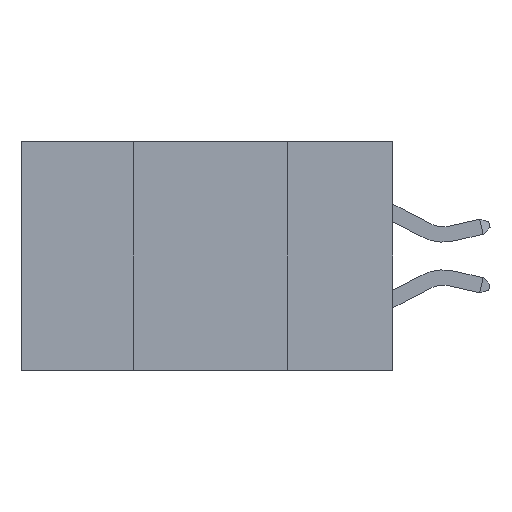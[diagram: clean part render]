
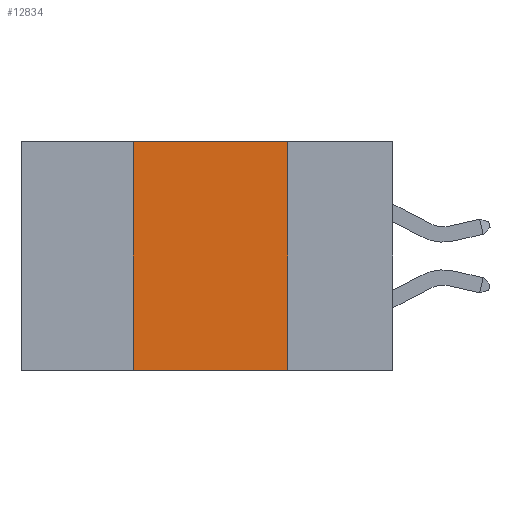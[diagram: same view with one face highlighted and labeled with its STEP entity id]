
A CAD part, left-side view. The second image highlights one B-rep face of the part: STEP entity #12834.
In plain terms, the highlighted planar face has unit normal (-1, 0, 0).
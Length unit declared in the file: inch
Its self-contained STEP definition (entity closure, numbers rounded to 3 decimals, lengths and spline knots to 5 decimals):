
#938 = ORIENTED_EDGE ( 'NONE', *, *, #9733, .T. ) ;
#943 = VECTOR ( 'NONE', #3581, 39.37008 ) ;
#1372 = CARTESIAN_POINT ( 'NONE',  ( 0., 0.6, 0. ) ) ;
#1464 = EDGE_CURVE ( 'NONE', #2867, #10343, #8704, .T. ) ;
#2004 = CARTESIAN_POINT ( 'NONE',  ( 0., 0.42, 0. ) ) ;
#2183 = CARTESIAN_POINT ( 'NONE',  ( 0., 0.17, -0.37 ) ) ;
#2352 = FACE_OUTER_BOUND ( 'NONE', #7382, .T. ) ;
#2500 = ORIENTED_EDGE ( 'NONE', *, *, #11791, .F. ) ;
#2699 = CARTESIAN_POINT ( 'NONE',  ( 0., 0.42, -0.37 ) ) ;
#2747 = LINE ( 'NONE', #5435, #7604 ) ;
#2867 = VERTEX_POINT ( 'NONE', #2699 ) ;
#3130 = DIRECTION ( 'NONE',  ( 0., 0., 1. ) ) ;
#3300 = CARTESIAN_POINT ( 'NONE',  ( 0., 0.42, 0. ) ) ;
#3566 = CARTESIAN_POINT ( 'NONE',  ( 0., 0.17, 0. ) ) ;
#3581 = DIRECTION ( 'NONE',  ( 0., -1., 0. ) ) ;
#4274 = VERTEX_POINT ( 'NONE', #2183 ) ;
#5435 = CARTESIAN_POINT ( 'NONE',  ( 0., 0.6, -0.37 ) ) ;
#5662 = DIRECTION ( 'NONE',  ( 1., 0., 0. ) ) ;
#6876 = VECTOR ( 'NONE', #9038, 39.37008 ) ;
#7234 = LINE ( 'NONE', #10057, #6876 ) ;
#7382 = EDGE_LOOP ( 'NONE', ( #2500, #12063, #11759, #938 ) ) ;
#7604 = VECTOR ( 'NONE', #10760, 39.37008 ) ;
#7832 = PLANE ( 'NONE',  #11953 ) ;
#8704 = LINE ( 'NONE', #3300, #13708 ) ;
#9038 = DIRECTION ( 'NONE',  ( 0., 0., -1. ) ) ;
#9733 = EDGE_CURVE ( 'NONE', #2867, #4274, #2747, .T. ) ;
#10057 = CARTESIAN_POINT ( 'NONE',  ( 0., 0.17, 0. ) ) ;
#10343 = VERTEX_POINT ( 'NONE', #2004 ) ;
#10760 = DIRECTION ( 'NONE',  ( 0., -1., 0. ) ) ;
#11759 = ORIENTED_EDGE ( 'NONE', *, *, #1464, .F. ) ;
#11791 = EDGE_CURVE ( 'NONE', #11795, #4274, #7234, .T. ) ;
#11795 = VERTEX_POINT ( 'NONE', #3566 ) ;
#11953 = AXIS2_PLACEMENT_3D ( 'NONE', #11985, #5662, #12961 ) ;
#11985 = CARTESIAN_POINT ( 'NONE',  ( 0., 0.6, 0. ) ) ;
#12063 = ORIENTED_EDGE ( 'NONE', *, *, #12927, .F. ) ;
#12386 = LINE ( 'NONE', #1372, #943 ) ;
#12834 = ADVANCED_FACE ( 'NONE', ( #2352 ), #7832, .F. ) ;
#12927 = EDGE_CURVE ( 'NONE', #10343, #11795, #12386, .T. ) ;
#12961 = DIRECTION ( 'NONE',  ( 0., 0., -1. ) ) ;
#13708 = VECTOR ( 'NONE', #3130, 39.37008 ) ;
